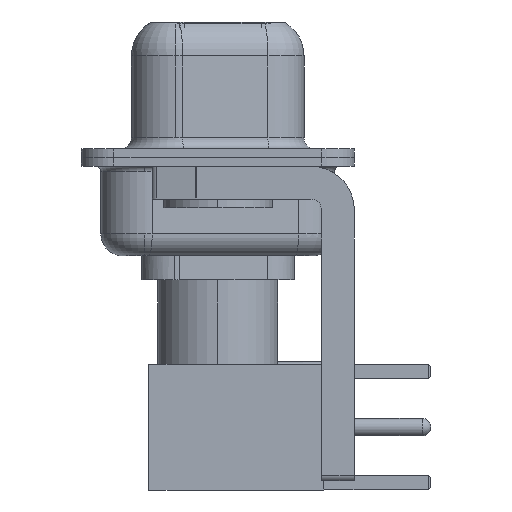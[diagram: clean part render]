
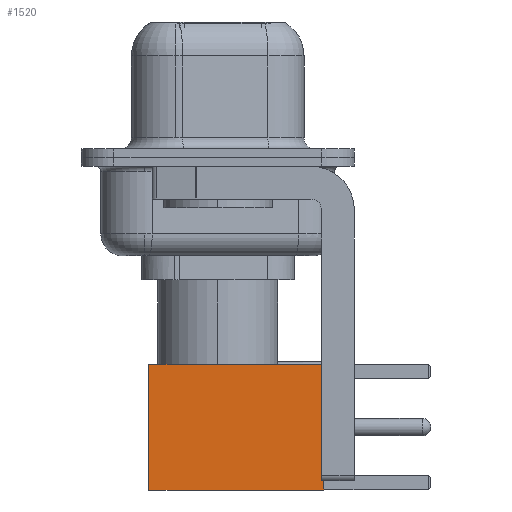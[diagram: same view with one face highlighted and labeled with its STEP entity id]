
A CAD part, left-side view. The second image highlights one B-rep face of the part: STEP entity #1520.
In plain terms, the highlighted face is planar.
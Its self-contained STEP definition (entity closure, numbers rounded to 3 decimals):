
#76 = VERTEX_POINT ( 'NONE', #27423 ) ;
#1073 = PLANE ( 'NONE',  #24983 ) ;
#1120 = VERTEX_POINT ( 'NONE', #10462 ) ;
#1231 = CARTESIAN_POINT ( 'NONE',  ( 2.875, 2.875, 0. ) ) ;
#1520 = ADVANCED_FACE ( 'NONE', ( #23789 ), #1073, .T. ) ;
#2694 = VECTOR ( 'NONE', #8075, 1000. ) ;
#4071 = ORIENTED_EDGE ( 'NONE', *, *, #23655, .T. ) ;
#4265 = ORIENTED_EDGE ( 'NONE', *, *, #10833, .F. ) ;
#5736 = DIRECTION ( 'NONE',  ( 0., 0., 1. ) ) ;
#6480 = CARTESIAN_POINT ( 'NONE',  ( 2.875, 2.875, 8. ) ) ;
#8075 = DIRECTION ( 'NONE',  ( -1., 0., 0. ) ) ;
#8295 = LINE ( 'NONE', #10073, #24335 ) ;
#8765 = LINE ( 'NONE', #13145, #12330 ) ;
#10073 = CARTESIAN_POINT ( 'NONE',  ( 2.875, 2.875, 0. ) ) ;
#10236 = VERTEX_POINT ( 'NONE', #11251 ) ;
#10417 = CARTESIAN_POINT ( 'NONE',  ( 0., 2.875, 8. ) ) ;
#10462 = CARTESIAN_POINT ( 'NONE',  ( 2.875, 2.875, 0. ) ) ;
#10833 = EDGE_CURVE ( 'NONE', #17708, #76, #17430, .T. ) ;
#11251 = CARTESIAN_POINT ( 'NONE',  ( -2.875, 2.875, 0. ) ) ;
#12330 = VECTOR ( 'NONE', #28433, 1000. ) ;
#13145 = CARTESIAN_POINT ( 'NONE',  ( 0., 2.875, 0. ) ) ;
#14543 = LINE ( 'NONE', #27629, #19018 ) ;
#14942 = ORIENTED_EDGE ( 'NONE', *, *, #22187, .F. ) ;
#16715 = ORIENTED_EDGE ( 'NONE', *, *, #17884, .T. ) ;
#17430 = LINE ( 'NONE', #10417, #2694 ) ;
#17708 = VERTEX_POINT ( 'NONE', #6480 ) ;
#17884 = EDGE_CURVE ( 'NONE', #1120, #10236, #8765, .T. ) ;
#19018 = VECTOR ( 'NONE', #20730, 1000. ) ;
#19924 = EDGE_LOOP ( 'NONE', ( #4071, #16715, #14942, #4265 ) ) ;
#20730 = DIRECTION ( 'NONE',  ( 0., 0., -1. ) ) ;
#22187 = EDGE_CURVE ( 'NONE', #76, #10236, #14543, .T. ) ;
#23488 = DIRECTION ( 'NONE',  ( 0., 1., 0. ) ) ;
#23655 = EDGE_CURVE ( 'NONE', #17708, #1120, #8295, .T. ) ;
#23789 = FACE_OUTER_BOUND ( 'NONE', #19924, .T. ) ;
#24335 = VECTOR ( 'NONE', #28405, 1000. ) ;
#24983 = AXIS2_PLACEMENT_3D ( 'NONE', #1231, #23488, #5736 ) ;
#27423 = CARTESIAN_POINT ( 'NONE',  ( -2.875, 2.875, 8. ) ) ;
#27629 = CARTESIAN_POINT ( 'NONE',  ( -2.875, 2.875, 0. ) ) ;
#28405 = DIRECTION ( 'NONE',  ( 0., 0., -1. ) ) ;
#28433 = DIRECTION ( 'NONE',  ( -1., 0., 0. ) ) ;
